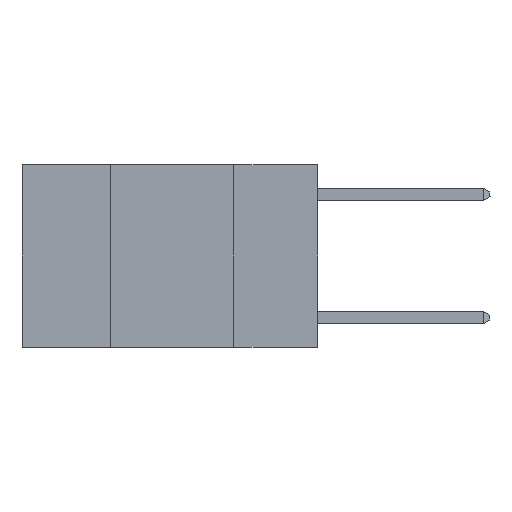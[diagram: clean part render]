
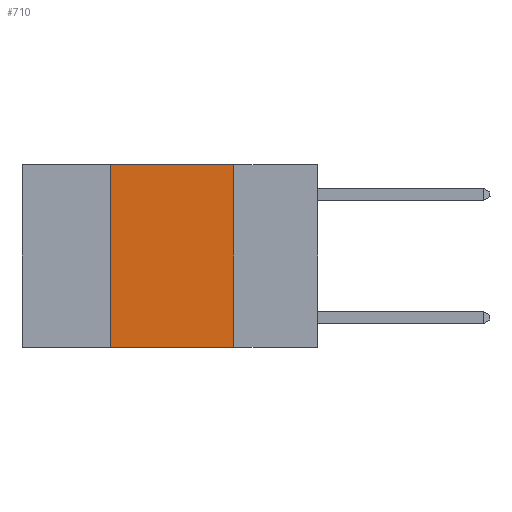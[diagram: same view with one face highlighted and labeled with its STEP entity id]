
A CAD part, left-side view. The second image highlights one B-rep face of the part: STEP entity #710.
In plain terms, the highlighted planar face has unit normal (-1, 0, 0).
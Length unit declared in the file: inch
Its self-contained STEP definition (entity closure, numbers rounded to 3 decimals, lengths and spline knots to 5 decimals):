
#76 = CARTESIAN_POINT ( 'NONE',  ( 0., 0.42, -0.37 ) ) ;
#710 = ADVANCED_FACE ( 'NONE', ( #1961 ), #1509, .F. ) ;
#890 = DIRECTION ( 'NONE',  ( 0., -1., 0. ) ) ;
#1021 = CARTESIAN_POINT ( 'NONE',  ( 0., 0.42, 0. ) ) ;
#1087 = CARTESIAN_POINT ( 'NONE',  ( 0., 0.42, 0. ) ) ;
#1509 = PLANE ( 'NONE',  #7573 ) ;
#1526 = EDGE_CURVE ( 'NONE', #7877, #8578, #4910, .T. ) ;
#1646 = DIRECTION ( 'NONE',  ( 0., 0., 1. ) ) ;
#1961 = FACE_OUTER_BOUND ( 'NONE', #5501, .T. ) ;
#2003 = VECTOR ( 'NONE', #5389, 39.37008 ) ;
#2124 = VECTOR ( 'NONE', #890, 39.37008 ) ;
#2125 = CARTESIAN_POINT ( 'NONE',  ( 0., 0.17, 0. ) ) ;
#2529 = ORIENTED_EDGE ( 'NONE', *, *, #10368, .F. ) ;
#2554 = CARTESIAN_POINT ( 'NONE',  ( 0., 0.6, 0. ) ) ;
#2772 = VERTEX_POINT ( 'NONE', #7154 ) ;
#3084 = CARTESIAN_POINT ( 'NONE',  ( 0., 0.17, -0.37 ) ) ;
#4293 = EDGE_CURVE ( 'NONE', #7877, #8294, #4583, .T. ) ;
#4583 = LINE ( 'NONE', #5018, #2124 ) ;
#4657 = ORIENTED_EDGE ( 'NONE', *, *, #4293, .T. ) ;
#4694 = DIRECTION ( 'NONE',  ( 0., 0., -1. ) ) ;
#4910 = LINE ( 'NONE', #1087, #8867 ) ;
#5018 = CARTESIAN_POINT ( 'NONE',  ( 0., 0.6, -0.37 ) ) ;
#5389 = DIRECTION ( 'NONE',  ( 0., 0., -1. ) ) ;
#5501 = EDGE_LOOP ( 'NONE', ( #2529, #9333, #5541, #4657 ) ) ;
#5541 = ORIENTED_EDGE ( 'NONE', *, *, #1526, .F. ) ;
#6350 = LINE ( 'NONE', #2125, #2003 ) ;
#7154 = CARTESIAN_POINT ( 'NONE',  ( 0., 0.17, 0. ) ) ;
#7573 = AXIS2_PLACEMENT_3D ( 'NONE', #10219, #8291, #4694 ) ;
#7721 = VECTOR ( 'NONE', #8234, 39.37008 ) ;
#7877 = VERTEX_POINT ( 'NONE', #76 ) ;
#7884 = EDGE_CURVE ( 'NONE', #8578, #2772, #9865, .T. ) ;
#8234 = DIRECTION ( 'NONE',  ( 0., -1., 0. ) ) ;
#8291 = DIRECTION ( 'NONE',  ( 1., 0., 0. ) ) ;
#8294 = VERTEX_POINT ( 'NONE', #3084 ) ;
#8578 = VERTEX_POINT ( 'NONE', #1021 ) ;
#8867 = VECTOR ( 'NONE', #1646, 39.37008 ) ;
#9333 = ORIENTED_EDGE ( 'NONE', *, *, #7884, .F. ) ;
#9865 = LINE ( 'NONE', #2554, #7721 ) ;
#10219 = CARTESIAN_POINT ( 'NONE',  ( 0., 0.6, 0. ) ) ;
#10368 = EDGE_CURVE ( 'NONE', #2772, #8294, #6350, .T. ) ;
